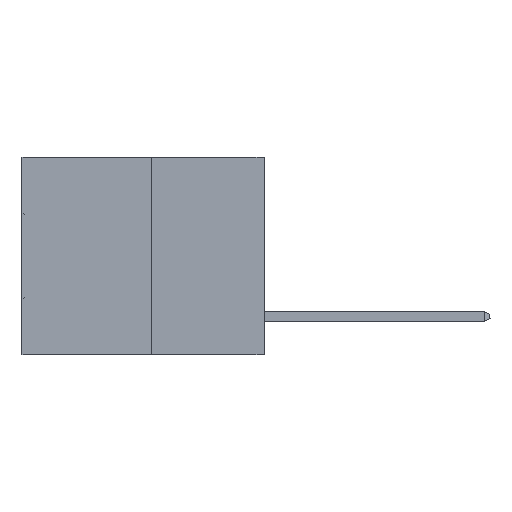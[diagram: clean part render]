
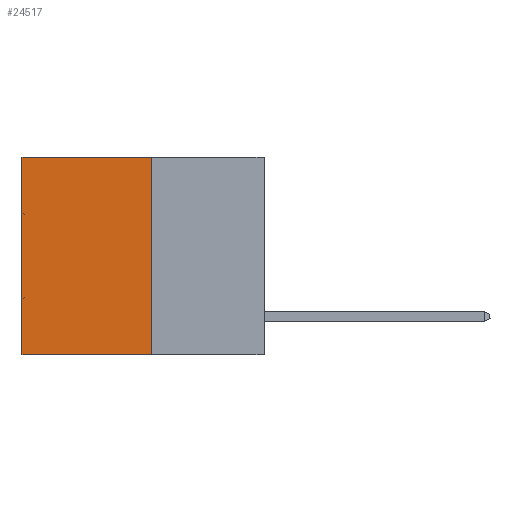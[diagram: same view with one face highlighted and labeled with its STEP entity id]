
A CAD part, left-side view. The second image highlights one B-rep face of the part: STEP entity #24517.
In plain terms, the highlighted planar face has unit normal (-1, 0, 0).
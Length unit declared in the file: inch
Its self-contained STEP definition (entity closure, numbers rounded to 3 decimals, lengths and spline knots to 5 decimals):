
#792 = CARTESIAN_POINT ( 'NONE',  ( 0.3165, 0.28, -0.49 ) ) ;
#1300 = VECTOR ( 'NONE', #3258, 39.37008 ) ;
#1775 = ORIENTED_EDGE ( 'NONE', *, *, #18432, .F. ) ;
#2600 = VECTOR ( 'NONE', #19655, 39.37008 ) ;
#3258 = DIRECTION ( 'NONE',  ( 0., 1., 0. ) ) ;
#3980 = DIRECTION ( 'NONE',  ( 0., 0., -1. ) ) ;
#4180 = LINE ( 'NONE', #20319, #19997 ) ;
#4494 = DIRECTION ( 'NONE',  ( 0., 0., -1. ) ) ;
#5724 = CARTESIAN_POINT ( 'NONE',  ( 0.3165, 0.28, 0. ) ) ;
#5766 = EDGE_CURVE ( 'NONE', #17761, #13652, #4180, .T. ) ;
#8935 = VERTEX_POINT ( 'NONE', #11444 ) ;
#9711 = CARTESIAN_POINT ( 'NONE',  ( 0.3165, 0.6, -0.49 ) ) ;
#10428 = ORIENTED_EDGE ( 'NONE', *, *, #5766, .T. ) ;
#10518 = AXIS2_PLACEMENT_3D ( 'NONE', #14661, #27918, #3980 ) ;
#11444 = CARTESIAN_POINT ( 'NONE',  ( 0.3165, 0.28, -0.49 ) ) ;
#11951 = CARTESIAN_POINT ( 'NONE',  ( 0.3165, 0.6, 0. ) ) ;
#12616 = ORIENTED_EDGE ( 'NONE', *, *, #23812, .F. ) ;
#13652 = VERTEX_POINT ( 'NONE', #9711 ) ;
#14661 = CARTESIAN_POINT ( 'NONE',  ( 0.3165, 0.28, -0.49 ) ) ;
#17466 = EDGE_CURVE ( 'NONE', #20995, #17761, #32508, .T. ) ;
#17761 = VERTEX_POINT ( 'NONE', #11951 ) ;
#18432 = EDGE_CURVE ( 'NONE', #8935, #13652, #26614, .T. ) ;
#19655 = DIRECTION ( 'NONE',  ( 0., 1., 0. ) ) ;
#19659 = PLANE ( 'NONE',  #10518 ) ;
#19822 = VECTOR ( 'NONE', #21687, 39.37008 ) ;
#19997 = VECTOR ( 'NONE', #4494, 39.37008 ) ;
#20319 = CARTESIAN_POINT ( 'NONE',  ( 0.3165, 0.6, -0.49 ) ) ;
#20649 = LINE ( 'NONE', #792, #19822 ) ;
#20995 = VERTEX_POINT ( 'NONE', #5724 ) ;
#21687 = DIRECTION ( 'NONE',  ( 0., 0., -1. ) ) ;
#22108 = CARTESIAN_POINT ( 'NONE',  ( 0.3165, 0.28, -0.49 ) ) ;
#22111 = CARTESIAN_POINT ( 'NONE',  ( 0.3165, 0.28, 0. ) ) ;
#23812 = EDGE_CURVE ( 'NONE', #20995, #8935, #20649, .T. ) ;
#23898 = FACE_OUTER_BOUND ( 'NONE', #31348, .T. ) ;
#24517 = ADVANCED_FACE ( 'NONE', ( #23898 ), #19659, .F. ) ;
#26614 = LINE ( 'NONE', #22108, #1300 ) ;
#27827 = ORIENTED_EDGE ( 'NONE', *, *, #17466, .T. ) ;
#27918 = DIRECTION ( 'NONE',  ( 1., 0., 0. ) ) ;
#31348 = EDGE_LOOP ( 'NONE', ( #10428, #1775, #12616, #27827 ) ) ;
#32508 = LINE ( 'NONE', #22111, #2600 ) ;
